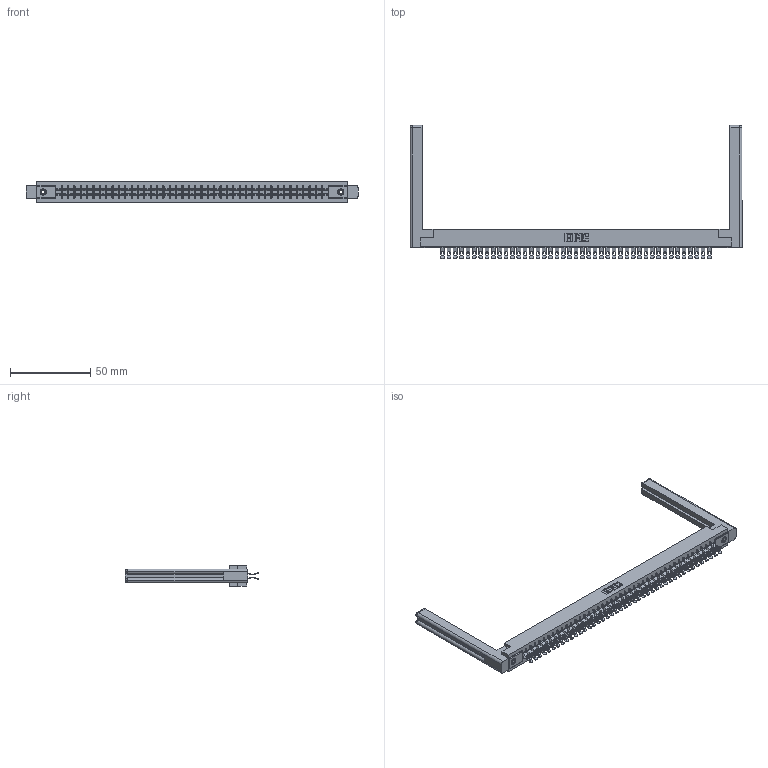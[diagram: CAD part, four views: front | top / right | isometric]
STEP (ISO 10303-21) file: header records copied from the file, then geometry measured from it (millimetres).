
FILE_DESCRIPTION (( 'STEP AP203' ), '1' );
FILE_NAME ('315-086-555-258.STEP', '2019-09-11T00:24:01', ( '' ), ( '' ), 'SwSTEP 2.0', 'SolidWorks 2016', '' );
FILE_SCHEMA (( 'CONFIG_CONTROL_DESIGN' ));
Length unit declared in the file: inch
Products named in the file (5): 315-086-555-258; 307-220-058; 305-290-001_555; 345-250-001_345-250-001-102; 305 Part_.156 Dia
Assembly tree (91 placements, depth 2):
  315-086-555-258
    305 Part_.156 Dia
    305-290-001_555  x86
    345-250-001_345-250-001-102  x2
    307-220-058  x2
Bounding box: 207.01 x 83.06 x 12.7 mm (x, y, z)
Volume: 29013.9 mm3; surface area: 34304.8 mm2
Topology: 91 solids, 91 shells, 5934 faces, 17655 edges, 11526 vertices
Faces by surface type: plane 2904, cylinder 2834, sphere 172, cone 12, torus 12
Entity records: 49693 total; most frequent: CARTESIAN_POINT 8256, ORIENTED_EDGE 8128, DIRECTION 7942, EDGE_CURVE 4064, LINE 3258, VECTOR 3258, VERTEX_POINT 2586, AXIS2_PLACEMENT_3D 2342
